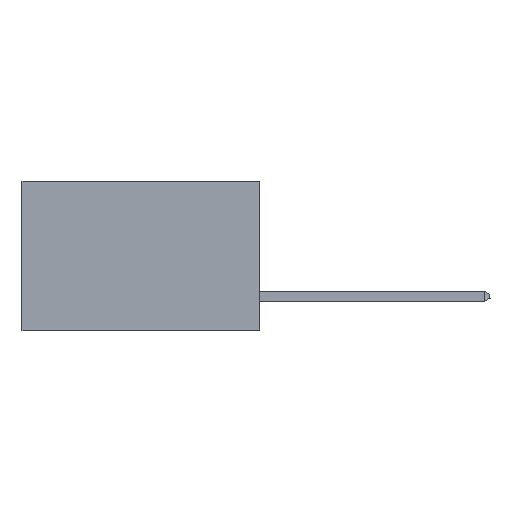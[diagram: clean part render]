
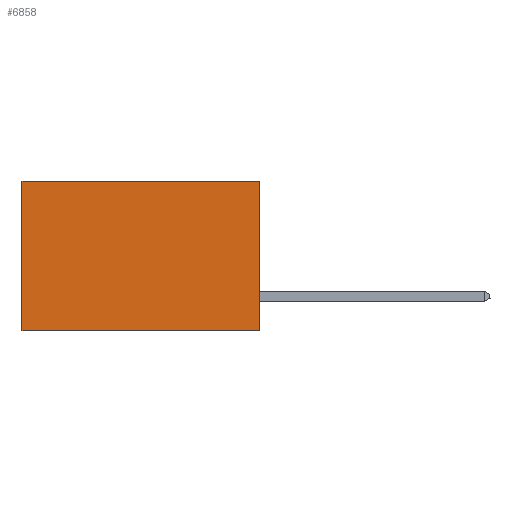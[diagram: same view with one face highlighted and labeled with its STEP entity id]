
A CAD part, left-side view. The second image highlights one B-rep face of the part: STEP entity #6858.
In plain terms, the highlighted planar face has unit normal (-1, 0, 0).
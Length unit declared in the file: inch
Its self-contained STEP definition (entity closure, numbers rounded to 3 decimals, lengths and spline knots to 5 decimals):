
#838 = EDGE_LOOP ( 'NONE', ( #3114, #4472, #18728, #4495 ) ) ;
#845 = CARTESIAN_POINT ( 'NONE',  ( 0.277, 0., 0. ) ) ;
#1105 = VECTOR ( 'NONE', #3602, 39.37008 ) ;
#1635 = LINE ( 'NONE', #7354, #5565 ) ;
#1961 = VECTOR ( 'NONE', #5976, 39.37008 ) ;
#2614 = EDGE_CURVE ( 'NONE', #18342, #13388, #16374, .T. ) ;
#3114 = ORIENTED_EDGE ( 'NONE', *, *, #9104, .T. ) ;
#3185 = CARTESIAN_POINT ( 'NONE',  ( 0.277, 0.59, 0. ) ) ;
#3602 = DIRECTION ( 'NONE',  ( 0., 1., 0. ) ) ;
#3957 = VECTOR ( 'NONE', #6610, 39.37008 ) ;
#4472 = ORIENTED_EDGE ( 'NONE', *, *, #6861, .F. ) ;
#4495 = ORIENTED_EDGE ( 'NONE', *, *, #2614, .T. ) ;
#4897 = CARTESIAN_POINT ( 'NONE',  ( 0.277, 0., -0.37 ) ) ;
#5565 = VECTOR ( 'NONE', #7285, 39.37008 ) ;
#5976 = DIRECTION ( 'NONE',  ( 0., 0., -1. ) ) ;
#5999 = CARTESIAN_POINT ( 'NONE',  ( 0.277, 0.59, -0.37 ) ) ;
#6610 = DIRECTION ( 'NONE',  ( 0., 0., -1. ) ) ;
#6858 = ADVANCED_FACE ( 'NONE', ( #10056 ), #7804, .F. ) ;
#6861 = EDGE_CURVE ( 'NONE', #9251, #17611, #1635, .T. ) ;
#7285 = DIRECTION ( 'NONE',  ( 0., 1., 0. ) ) ;
#7354 = CARTESIAN_POINT ( 'NONE',  ( 0.277, 0., -0.37 ) ) ;
#7523 = DIRECTION ( 'NONE',  ( 0., 0., -1. ) ) ;
#7548 = DIRECTION ( 'NONE',  ( 1., 0., 0. ) ) ;
#7586 = CARTESIAN_POINT ( 'NONE',  ( 0.277, 0., -0.37 ) ) ;
#7804 = PLANE ( 'NONE',  #17763 ) ;
#9104 = EDGE_CURVE ( 'NONE', #13388, #17611, #17644, .T. ) ;
#9163 = CARTESIAN_POINT ( 'NONE',  ( 0.277, 0., 0. ) ) ;
#9251 = VERTEX_POINT ( 'NONE', #4897 ) ;
#10056 = FACE_OUTER_BOUND ( 'NONE', #838, .T. ) ;
#13388 = VERTEX_POINT ( 'NONE', #3185 ) ;
#14245 = EDGE_CURVE ( 'NONE', #18342, #9251, #15802, .T. ) ;
#15433 = CARTESIAN_POINT ( 'NONE',  ( 0.277, 0., -0.37 ) ) ;
#15802 = LINE ( 'NONE', #15433, #3957 ) ;
#16374 = LINE ( 'NONE', #845, #1105 ) ;
#17611 = VERTEX_POINT ( 'NONE', #18964 ) ;
#17644 = LINE ( 'NONE', #5999, #1961 ) ;
#17763 = AXIS2_PLACEMENT_3D ( 'NONE', #7586, #7548, #7523 ) ;
#18342 = VERTEX_POINT ( 'NONE', #9163 ) ;
#18728 = ORIENTED_EDGE ( 'NONE', *, *, #14245, .F. ) ;
#18964 = CARTESIAN_POINT ( 'NONE',  ( 0.277, 0.59, -0.37 ) ) ;
